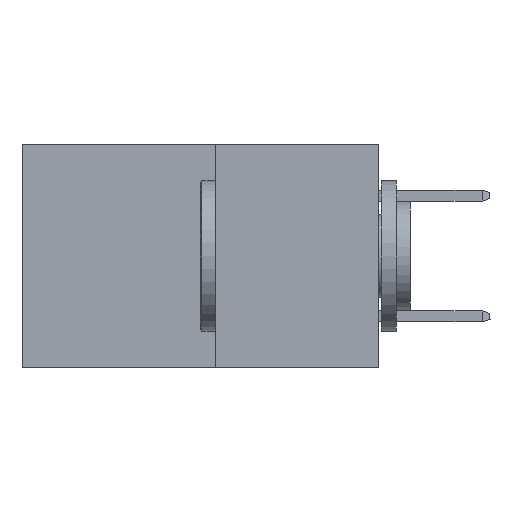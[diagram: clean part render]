
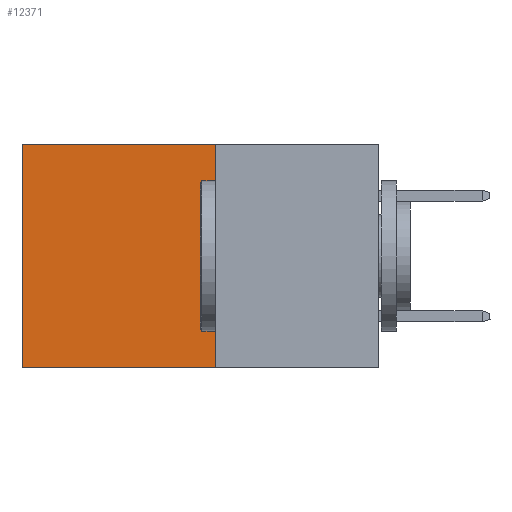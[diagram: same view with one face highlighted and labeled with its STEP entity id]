
A CAD part, left-side view. The second image highlights one B-rep face of the part: STEP entity #12371.
In plain terms, the highlighted planar face has unit normal (-1, 0, 0).
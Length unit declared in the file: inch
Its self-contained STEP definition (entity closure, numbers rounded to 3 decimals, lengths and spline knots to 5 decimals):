
#164 = ORIENTED_EDGE ( 'NONE', *, *, #2344, .T. ) ;
#193 = EDGE_CURVE ( 'NONE', #21014, #4565, #10679, .T. ) ;
#475 = DIRECTION ( 'NONE',  ( 0., 0., -1. ) ) ;
#906 = DIRECTION ( 'NONE',  ( 0., 1., 0. ) ) ;
#914 = CARTESIAN_POINT ( 'NONE',  ( 0.277, 0.27, 0. ) ) ;
#2231 = DIRECTION ( 'NONE',  ( 0., 0., -1. ) ) ;
#2344 = EDGE_CURVE ( 'NONE', #17877, #20245, #10200, .T. ) ;
#3809 = CARTESIAN_POINT ( 'NONE',  ( 0.277, 0.27, -0.37 ) ) ;
#4432 = LINE ( 'NONE', #24393, #22152 ) ;
#4565 = VERTEX_POINT ( 'NONE', #25064 ) ;
#7122 = ORIENTED_EDGE ( 'NONE', *, *, #193, .F. ) ;
#8518 = EDGE_CURVE ( 'NONE', #17877, #21014, #12313, .T. ) ;
#9982 = VECTOR ( 'NONE', #12542, 39.37008 ) ;
#10200 = LINE ( 'NONE', #914, #11591 ) ;
#10679 = LINE ( 'NONE', #3809, #9982 ) ;
#11534 = EDGE_CURVE ( 'NONE', #20245, #4565, #4432, .T. ) ;
#11591 = VECTOR ( 'NONE', #906, 39.37008 ) ;
#11622 = VECTOR ( 'NONE', #12335, 39.37008 ) ;
#11683 = PLANE ( 'NONE',  #23810 ) ;
#11875 = FACE_OUTER_BOUND ( 'NONE', #28616, .T. ) ;
#12313 = LINE ( 'NONE', #12620, #11622 ) ;
#12335 = DIRECTION ( 'NONE',  ( 0., 0., -1. ) ) ;
#12371 = ADVANCED_FACE ( 'NONE', ( #11875 ), #11683, .F. ) ;
#12542 = DIRECTION ( 'NONE',  ( 0., 1., 0. ) ) ;
#12620 = CARTESIAN_POINT ( 'NONE',  ( 0.277, 0.27, -0.37 ) ) ;
#13936 = DIRECTION ( 'NONE',  ( 1., 0., 0. ) ) ;
#17453 = CARTESIAN_POINT ( 'NONE',  ( 0.277, 0.27, 0. ) ) ;
#17877 = VERTEX_POINT ( 'NONE', #17453 ) ;
#17889 = CARTESIAN_POINT ( 'NONE',  ( 0.277, 0.59, 0. ) ) ;
#18640 = CARTESIAN_POINT ( 'NONE',  ( 0.277, 0.27, -0.37 ) ) ;
#20245 = VERTEX_POINT ( 'NONE', #17889 ) ;
#21014 = VERTEX_POINT ( 'NONE', #18640 ) ;
#22152 = VECTOR ( 'NONE', #2231, 39.37008 ) ;
#23386 = ORIENTED_EDGE ( 'NONE', *, *, #8518, .F. ) ;
#23810 = AXIS2_PLACEMENT_3D ( 'NONE', #27011, #13936, #475 ) ;
#24393 = CARTESIAN_POINT ( 'NONE',  ( 0.277, 0.59, -0.37 ) ) ;
#25064 = CARTESIAN_POINT ( 'NONE',  ( 0.277, 0.59, -0.37 ) ) ;
#27011 = CARTESIAN_POINT ( 'NONE',  ( 0.277, 0.27, -0.37 ) ) ;
#27024 = ORIENTED_EDGE ( 'NONE', *, *, #11534, .T. ) ;
#28616 = EDGE_LOOP ( 'NONE', ( #27024, #7122, #23386, #164 ) ) ;
